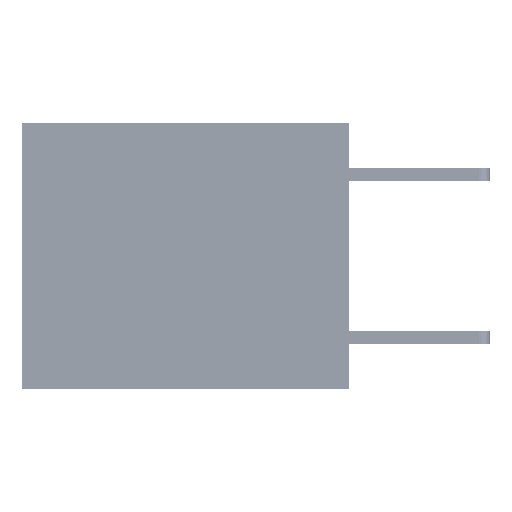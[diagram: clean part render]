
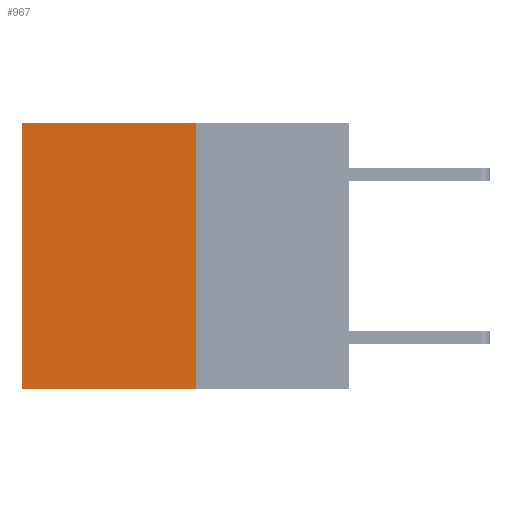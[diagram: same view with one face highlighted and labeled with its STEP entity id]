
A CAD part, left-side view. The second image highlights one B-rep face of the part: STEP entity #967.
In plain terms, the highlighted planar face has unit normal (-1, 0, 0).
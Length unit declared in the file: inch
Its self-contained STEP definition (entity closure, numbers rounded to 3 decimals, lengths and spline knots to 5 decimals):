
#12 = AXIS2_PLACEMENT_3D ( 'NONE', #20802, #12346, #33973 ) ;
#967 = ADVANCED_FACE ( 'NONE', ( #1705 ), #1417, .F. ) ;
#1417 = PLANE ( 'NONE',  #12 ) ;
#1705 = FACE_OUTER_BOUND ( 'NONE', #9595, .T. ) ;
#3161 = DIRECTION ( 'NONE',  ( 0., 0., -1. ) ) ;
#3562 = LINE ( 'NONE', #32918, #9556 ) ;
#3654 = VECTOR ( 'NONE', #21971, 39.37008 ) ;
#4581 = EDGE_CURVE ( 'NONE', #21081, #17570, #3562, .T. ) ;
#5465 = CARTESIAN_POINT ( 'NONE',  ( 0.3165, 0.6, 0. ) ) ;
#5943 = DIRECTION ( 'NONE',  ( 0., 1., 0. ) ) ;
#6411 = VECTOR ( 'NONE', #3161, 39.37008 ) ;
#8339 = LINE ( 'NONE', #16481, #3654 ) ;
#9044 = ORIENTED_EDGE ( 'NONE', *, *, #4581, .F. ) ;
#9556 = VECTOR ( 'NONE', #5943, 39.37008 ) ;
#9595 = EDGE_LOOP ( 'NONE', ( #22272, #9044, #17632, #14083 ) ) ;
#12346 = DIRECTION ( 'NONE',  ( 1., 0., 0. ) ) ;
#12672 = LINE ( 'NONE', #33325, #18607 ) ;
#14083 = ORIENTED_EDGE ( 'NONE', *, *, #23087, .T. ) ;
#14425 = VERTEX_POINT ( 'NONE', #31792 ) ;
#14723 = EDGE_CURVE ( 'NONE', #20734, #17570, #24665, .T. ) ;
#16481 = CARTESIAN_POINT ( 'NONE',  ( 0.3165, 0.28, -0.49 ) ) ;
#17015 = DIRECTION ( 'NONE',  ( 0., 1., 0. ) ) ;
#17017 = EDGE_CURVE ( 'NONE', #14425, #21081, #8339, .T. ) ;
#17570 = VERTEX_POINT ( 'NONE', #35080 ) ;
#17632 = ORIENTED_EDGE ( 'NONE', *, *, #17017, .F. ) ;
#18607 = VECTOR ( 'NONE', #17015, 39.37008 ) ;
#19221 = CARTESIAN_POINT ( 'NONE',  ( 0.3165, 0.6, -0.49 ) ) ;
#20734 = VERTEX_POINT ( 'NONE', #5465 ) ;
#20802 = CARTESIAN_POINT ( 'NONE',  ( 0.3165, 0.28, -0.49 ) ) ;
#21081 = VERTEX_POINT ( 'NONE', #35008 ) ;
#21971 = DIRECTION ( 'NONE',  ( 0., 0., -1. ) ) ;
#22272 = ORIENTED_EDGE ( 'NONE', *, *, #14723, .T. ) ;
#23087 = EDGE_CURVE ( 'NONE', #14425, #20734, #12672, .T. ) ;
#24665 = LINE ( 'NONE', #19221, #6411 ) ;
#31792 = CARTESIAN_POINT ( 'NONE',  ( 0.3165, 0.28, 0. ) ) ;
#32918 = CARTESIAN_POINT ( 'NONE',  ( 0.3165, 0.28, -0.49 ) ) ;
#33325 = CARTESIAN_POINT ( 'NONE',  ( 0.3165, 0.28, 0. ) ) ;
#33973 = DIRECTION ( 'NONE',  ( 0., 0., -1. ) ) ;
#35008 = CARTESIAN_POINT ( 'NONE',  ( 0.3165, 0.28, -0.49 ) ) ;
#35080 = CARTESIAN_POINT ( 'NONE',  ( 0.3165, 0.6, -0.49 ) ) ;
